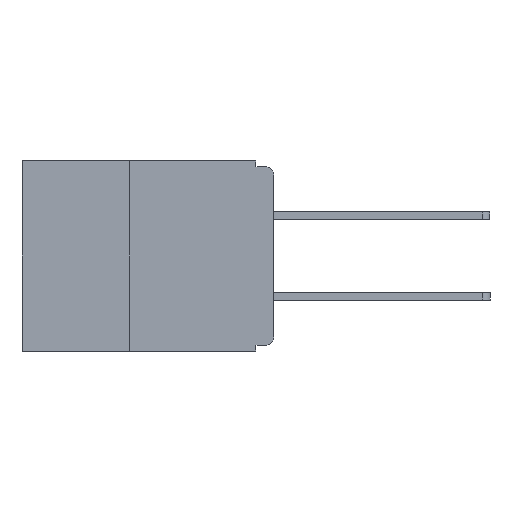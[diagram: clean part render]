
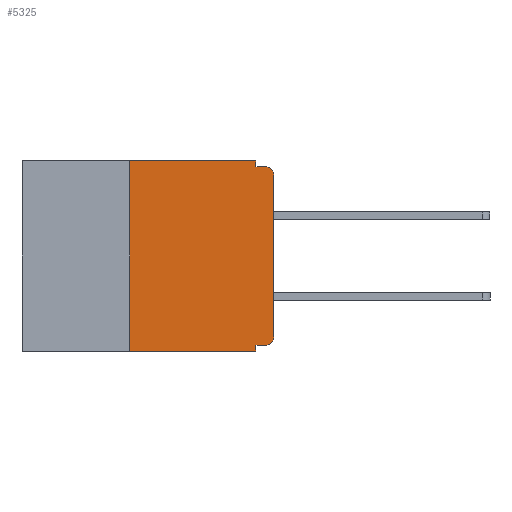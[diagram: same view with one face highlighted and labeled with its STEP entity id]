
A CAD part, left-side view. The second image highlights one B-rep face of the part: STEP entity #5325.
In plain terms, the highlighted planar face has unit normal (-1, 0, 0).
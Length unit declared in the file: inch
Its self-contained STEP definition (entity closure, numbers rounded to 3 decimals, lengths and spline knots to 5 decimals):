
#180 = VERTEX_POINT ( 'NONE', #25899 ) ;
#1032 = CIRCLE ( 'NONE', #23579, 0.015 ) ;
#1292 = VERTEX_POINT ( 'NONE', #13535 ) ;
#2370 = FACE_OUTER_BOUND ( 'NONE', #23576, .T. ) ;
#2807 = VECTOR ( 'NONE', #7199, 39.37008 ) ;
#3204 = LINE ( 'NONE', #19432, #9803 ) ;
#3355 = ORIENTED_EDGE ( 'NONE', *, *, #20018, .F. ) ;
#3692 = VERTEX_POINT ( 'NONE', #17034 ) ;
#3880 = CARTESIAN_POINT ( 'NONE',  ( 0., 0.031, -0.33 ) ) ;
#4109 = ORIENTED_EDGE ( 'NONE', *, *, #21646, .T. ) ;
#5325 = ADVANCED_FACE ( 'NONE', ( #2370 ), #22023, .F. ) ;
#5805 = VERTEX_POINT ( 'NONE', #15702 ) ;
#6356 = DIRECTION ( 'NONE',  ( 0., 0., 1. ) ) ;
#7196 = ORIENTED_EDGE ( 'NONE', *, *, #21088, .F. ) ;
#7199 = DIRECTION ( 'NONE',  ( 0., 0., -1. ) ) ;
#7627 = DIRECTION ( 'NONE',  ( -1., 0., 0. ) ) ;
#8533 = CARTESIAN_POINT ( 'NONE',  ( 0., 0., -0.32 ) ) ;
#8729 = DIRECTION ( 'NONE',  ( 0., 0., -1. ) ) ;
#8953 = ORIENTED_EDGE ( 'NONE', *, *, #27325, .F. ) ;
#9592 = CARTESIAN_POINT ( 'NONE',  ( 0., 0.25, 0. ) ) ;
#9803 = VECTOR ( 'NONE', #6356, 39.37008 ) ;
#10231 = CARTESIAN_POINT ( 'NONE',  ( 0., 0., -0.305 ) ) ;
#10364 = DIRECTION ( 'NONE',  ( 0., -1., 0. ) ) ;
#10786 = AXIS2_PLACEMENT_3D ( 'NONE', #26103, #13327, #8729 ) ;
#11275 = EDGE_CURVE ( 'NONE', #13432, #14504, #25938, .T. ) ;
#11879 = VECTOR ( 'NONE', #12588, 39.37008 ) ;
#12268 = ORIENTED_EDGE ( 'NONE', *, *, #15692, .T. ) ;
#12588 = DIRECTION ( 'NONE',  ( 0., 0., 1. ) ) ;
#13209 = ORIENTED_EDGE ( 'NONE', *, *, #24295, .F. ) ;
#13327 = DIRECTION ( 'NONE',  ( -1., 0., 0. ) ) ;
#13432 = VERTEX_POINT ( 'NONE', #21131 ) ;
#13501 = ORIENTED_EDGE ( 'NONE', *, *, #15900, .T. ) ;
#13535 = CARTESIAN_POINT ( 'NONE',  ( 0., 0.25, -0.33 ) ) ;
#14504 = VERTEX_POINT ( 'NONE', #3880 ) ;
#14546 = ORIENTED_EDGE ( 'NONE', *, *, #19377, .F. ) ;
#14743 = CARTESIAN_POINT ( 'NONE',  ( 0., 0.437, -0.33 ) ) ;
#14848 = VERTEX_POINT ( 'NONE', #9592 ) ;
#14937 = VECTOR ( 'NONE', #16606, 39.37008 ) ;
#15072 = VECTOR ( 'NONE', #16681, 39.37008 ) ;
#15272 = CIRCLE ( 'NONE', #10786, 0.015 ) ;
#15692 = EDGE_CURVE ( 'NONE', #1292, #14504, #19335, .T. ) ;
#15702 = CARTESIAN_POINT ( 'NONE',  ( 0., 0.015, -0.32 ) ) ;
#15709 = ORIENTED_EDGE ( 'NONE', *, *, #11275, .F. ) ;
#15900 = EDGE_CURVE ( 'NONE', #5805, #23794, #15272, .T. ) ;
#16606 = DIRECTION ( 'NONE',  ( 0., -1., 0. ) ) ;
#16681 = DIRECTION ( 'NONE',  ( 0., 0., -1. ) ) ;
#17034 = CARTESIAN_POINT ( 'NONE',  ( 0., 0.031, -0.01 ) ) ;
#17658 = LINE ( 'NONE', #27561, #11879 ) ;
#17770 = VERTEX_POINT ( 'NONE', #20055 ) ;
#18073 = CARTESIAN_POINT ( 'NONE',  ( 0., 0.031, -0.33 ) ) ;
#19335 = LINE ( 'NONE', #14743, #20662 ) ;
#19377 = EDGE_CURVE ( 'NONE', #14848, #27321, #26685, .T. ) ;
#19432 = CARTESIAN_POINT ( 'NONE',  ( 0., 0.25, -0.33 ) ) ;
#20018 = EDGE_CURVE ( 'NONE', #1292, #14848, #3204, .T. ) ;
#20055 = CARTESIAN_POINT ( 'NONE',  ( 0., 0., -0.025 ) ) ;
#20141 = ORIENTED_EDGE ( 'NONE', *, *, #20573, .T. ) ;
#20573 = EDGE_CURVE ( 'NONE', #23794, #17770, #17658, .T. ) ;
#20642 = CARTESIAN_POINT ( 'NONE',  ( 0., 0.015, -0.025 ) ) ;
#20647 = LINE ( 'NONE', #23015, #14937 ) ;
#20662 = VECTOR ( 'NONE', #27509, 39.37008 ) ;
#20781 = LINE ( 'NONE', #23168, #15072 ) ;
#20846 = AXIS2_PLACEMENT_3D ( 'NONE', #21854, #21825, #21801 ) ;
#21088 = EDGE_CURVE ( 'NONE', #3692, #180, #20647, .T. ) ;
#21131 = CARTESIAN_POINT ( 'NONE',  ( 0., 0.031, -0.32 ) ) ;
#21152 = CARTESIAN_POINT ( 'NONE',  ( 0., 0.437, 0. ) ) ;
#21419 = VECTOR ( 'NONE', #23831, 39.37008 ) ;
#21604 = CARTESIAN_POINT ( 'NONE',  ( 0., 0.031, 0. ) ) ;
#21646 = EDGE_CURVE ( 'NONE', #17770, #180, #1032, .T. ) ;
#21801 = DIRECTION ( 'NONE',  ( 0., 0., -1. ) ) ;
#21825 = DIRECTION ( 'NONE',  ( 1., 0., 0. ) ) ;
#21854 = CARTESIAN_POINT ( 'NONE',  ( 0., 0.437, 0. ) ) ;
#22023 = PLANE ( 'NONE',  #20846 ) ;
#22798 = DIRECTION ( 'NONE',  ( 0., 0., -1. ) ) ;
#23015 = CARTESIAN_POINT ( 'NONE',  ( 0., 0., -0.01 ) ) ;
#23168 = CARTESIAN_POINT ( 'NONE',  ( 0., 0.031, 0. ) ) ;
#23576 = EDGE_LOOP ( 'NONE', ( #20141, #4109, #7196, #13209, #14546, #3355, #12268, #15709, #8953, #13501 ) ) ;
#23579 = AXIS2_PLACEMENT_3D ( 'NONE', #20642, #7627, #22798 ) ;
#23794 = VERTEX_POINT ( 'NONE', #10231 ) ;
#23831 = DIRECTION ( 'NONE',  ( 0., 1., 0. ) ) ;
#24295 = EDGE_CURVE ( 'NONE', #27321, #3692, #20781, .T. ) ;
#25899 = CARTESIAN_POINT ( 'NONE',  ( 0., 0.015, -0.01 ) ) ;
#25938 = LINE ( 'NONE', #18073, #2807 ) ;
#26014 = VECTOR ( 'NONE', #10364, 39.37008 ) ;
#26103 = CARTESIAN_POINT ( 'NONE',  ( 0., 0.015, -0.305 ) ) ;
#26685 = LINE ( 'NONE', #21152, #26014 ) ;
#27068 = LINE ( 'NONE', #8533, #21419 ) ;
#27321 = VERTEX_POINT ( 'NONE', #21604 ) ;
#27325 = EDGE_CURVE ( 'NONE', #5805, #13432, #27068, .T. ) ;
#27509 = DIRECTION ( 'NONE',  ( 0., -1., 0. ) ) ;
#27561 = CARTESIAN_POINT ( 'NONE',  ( 0., 0., 0. ) ) ;
